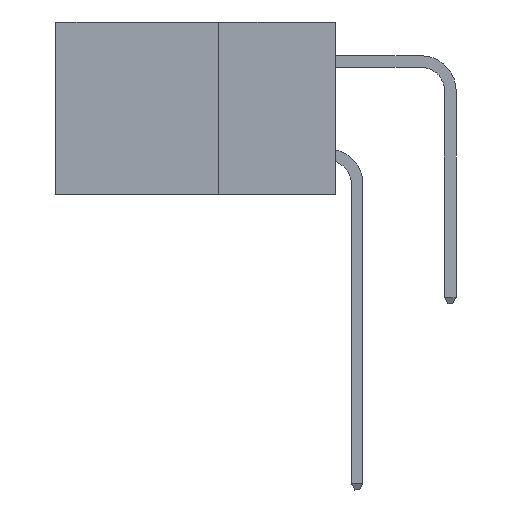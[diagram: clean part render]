
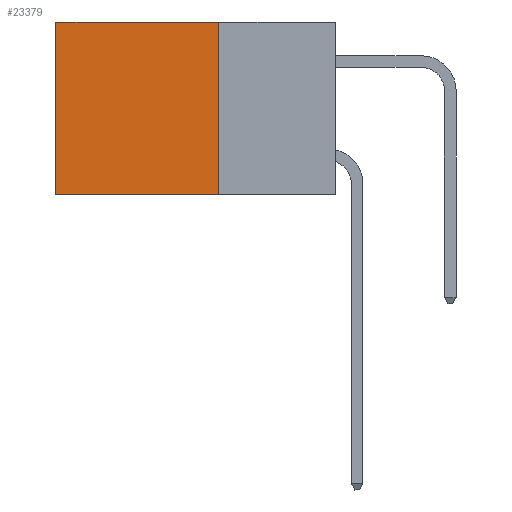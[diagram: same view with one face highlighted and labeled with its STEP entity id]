
A CAD part, left-side view. The second image highlights one B-rep face of the part: STEP entity #23379.
In plain terms, the highlighted planar face has unit normal (-1, 0, 0).
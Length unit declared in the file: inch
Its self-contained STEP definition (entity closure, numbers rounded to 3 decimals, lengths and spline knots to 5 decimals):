
#446 = LINE ( 'NONE', #3876, #23508 ) ;
#590 = CARTESIAN_POINT ( 'NONE',  ( 0.2875, 0.25, 0. ) ) ;
#2225 = VECTOR ( 'NONE', #18694, 39.37008 ) ;
#3179 = CARTESIAN_POINT ( 'NONE',  ( 0.2875, 0.25, 0. ) ) ;
#3637 = ORIENTED_EDGE ( 'NONE', *, *, #10605, .T. ) ;
#3876 = CARTESIAN_POINT ( 'NONE',  ( 0.2875, 0.25, 0. ) ) ;
#3956 = EDGE_CURVE ( 'NONE', #10899, #10515, #446, .T. ) ;
#4402 = DIRECTION ( 'NONE',  ( 0., 0., -1. ) ) ;
#4566 = VERTEX_POINT ( 'NONE', #26036 ) ;
#5926 = VERTEX_POINT ( 'NONE', #6354 ) ;
#6064 = DIRECTION ( 'NONE',  ( 0., 0., -1. ) ) ;
#6354 = CARTESIAN_POINT ( 'NONE',  ( 0.2875, 0.6, -0.37 ) ) ;
#7164 = ORIENTED_EDGE ( 'NONE', *, *, #3956, .T. ) ;
#7914 = AXIS2_PLACEMENT_3D ( 'NONE', #26201, #8138, #6064 ) ;
#8138 = DIRECTION ( 'NONE',  ( 1., 0., 0. ) ) ;
#9249 = EDGE_CURVE ( 'NONE', #10899, #4566, #11360, .T. ) ;
#10040 = EDGE_CURVE ( 'NONE', #4566, #5926, #18249, .T. ) ;
#10515 = VERTEX_POINT ( 'NONE', #12853 ) ;
#10578 = DIRECTION ( 'NONE',  ( 0., 1., 0. ) ) ;
#10605 = EDGE_CURVE ( 'NONE', #10515, #5926, #14165, .T. ) ;
#10899 = VERTEX_POINT ( 'NONE', #590 ) ;
#11360 = LINE ( 'NONE', #3179, #25691 ) ;
#11724 = VECTOR ( 'NONE', #4402, 39.37008 ) ;
#12853 = CARTESIAN_POINT ( 'NONE',  ( 0.2875, 0.6, 0. ) ) ;
#13162 = CARTESIAN_POINT ( 'NONE',  ( 0.2875, 0.6, 0. ) ) ;
#14035 = EDGE_LOOP ( 'NONE', ( #3637, #28016, #27707, #7164 ) ) ;
#14165 = LINE ( 'NONE', #13162, #11724 ) ;
#15391 = FACE_OUTER_BOUND ( 'NONE', #14035, .T. ) ;
#18249 = LINE ( 'NONE', #23094, #2225 ) ;
#18694 = DIRECTION ( 'NONE',  ( 0., 1., 0. ) ) ;
#19275 = DIRECTION ( 'NONE',  ( 0., 0., -1. ) ) ;
#19437 = PLANE ( 'NONE',  #7914 ) ;
#23094 = CARTESIAN_POINT ( 'NONE',  ( 0.2875, 0.25, -0.37 ) ) ;
#23379 = ADVANCED_FACE ( 'NONE', ( #15391 ), #19437, .F. ) ;
#23508 = VECTOR ( 'NONE', #10578, 39.37008 ) ;
#25691 = VECTOR ( 'NONE', #19275, 39.37008 ) ;
#26036 = CARTESIAN_POINT ( 'NONE',  ( 0.2875, 0.25, -0.37 ) ) ;
#26201 = CARTESIAN_POINT ( 'NONE',  ( 0.2875, 0.25, 0. ) ) ;
#27707 = ORIENTED_EDGE ( 'NONE', *, *, #9249, .F. ) ;
#28016 = ORIENTED_EDGE ( 'NONE', *, *, #10040, .F. ) ;
